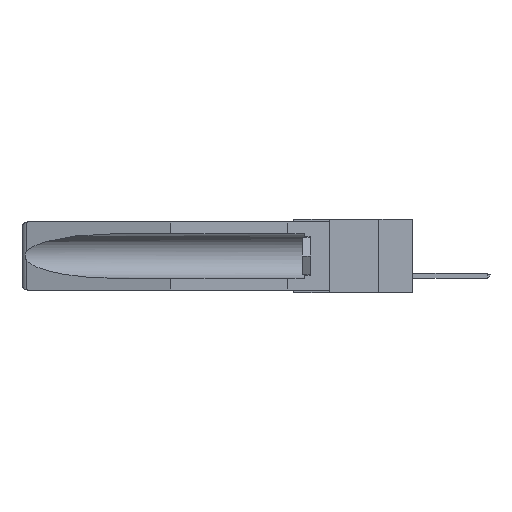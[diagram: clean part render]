
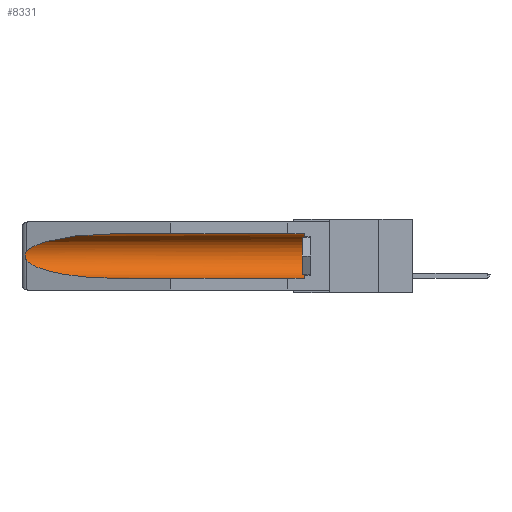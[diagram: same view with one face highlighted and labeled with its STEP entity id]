
A CAD part, left-side view. The second image highlights one B-rep face of the part: STEP entity #8331.
In plain terms, the highlighted cylindrical face has radius 2.857 mm (diameter 5.715 mm), a partial arc.
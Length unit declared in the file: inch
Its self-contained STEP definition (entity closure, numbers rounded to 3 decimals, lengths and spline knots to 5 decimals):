
#1018 = CARTESIAN_POINT ( 'NONE',  ( 0.155, 0.126, -0.284 ) ) ;
#1544 =( BOUNDED_CURVE ( )  B_SPLINE_CURVE ( 3, ( #12412, #15282, #9907, #25426 ),
 .UNSPECIFIED., .F., .F. ) 
 B_SPLINE_CURVE_WITH_KNOTS ( ( 4, 4 ),
 ( 0.1948, 1.5708 ),
 .UNSPECIFIED. ) 
 CURVE ( )  GEOMETRIC_REPRESENTATION_ITEM ( )  RATIONAL_B_SPLINE_CURVE ( ( 1., 0.848, 0.848, 1. ) ) 
 REPRESENTATION_ITEM ( '' )  );
#1725 = CARTESIAN_POINT ( 'NONE',  ( 0.26537, 1.52718, -0.14972 ) ) ;
#3282 = CYLINDRICAL_SURFACE ( 'NONE', #5432, 0.1125 ) ;
#3597 = VERTEX_POINT ( 'NONE', #26638 ) ;
#4484 = DIRECTION ( 'NONE',  ( 0., 0., 1. ) ) ;
#4537 = CARTESIAN_POINT ( 'NONE',  ( 0.2673, 1.5327, -0.16383 ) ) ;
#5125 = VERTEX_POINT ( 'NONE', #1018 ) ;
#5432 = AXIS2_PLACEMENT_3D ( 'NONE', #12078, #9359, #4484 ) ;
#6015 = ORIENTED_EDGE ( 'NONE', *, *, #29916, .T. ) ;
#6448 = CARTESIAN_POINT ( 'NONE',  ( 0.26537, 1.52718, -0.19328 ) ) ;
#7262 = CIRCLE ( 'NONE', #9602, 0.1125 ) ;
#8078 = LINE ( 'NONE', #31128, #20092 ) ;
#8331 = ADVANCED_FACE ( 'NONE', ( #16072 ), #3282, .F. ) ;
#8594 = VERTEX_POINT ( 'NONE', #15827 ) ;
#8678 = EDGE_LOOP ( 'NONE', ( #13634, #25850, #21183, #23184, #6015, #9770 ) ) ;
#9359 = DIRECTION ( 'NONE',  ( 0., 1., 0. ) ) ;
#9602 = AXIS2_PLACEMENT_3D ( 'NONE', #24450, #14224, #14333 ) ;
#9770 = ORIENTED_EDGE ( 'NONE', *, *, #11382, .T. ) ;
#9907 = CARTESIAN_POINT ( 'NONE',  ( 0.21114, 1.30732, -0.284 ) ) ;
#10017 = VERTEX_POINT ( 'NONE', #33198 ) ;
#11382 = EDGE_CURVE ( 'NONE', #27803, #10017, #25628, .T. ) ;
#12078 = CARTESIAN_POINT ( 'NONE',  ( 0.155, -0.30754, -0.1715 ) ) ;
#12137 = CARTESIAN_POINT ( 'NONE',  ( 0.2675, 1.53308, -0.16763 ) ) ;
#12375 = VERTEX_POINT ( 'NONE', #6448 ) ;
#12412 = CARTESIAN_POINT ( 'NONE',  ( 0.26537, 1.52718, -0.19328 ) ) ;
#13436 = B_SPLINE_CURVE_WITH_KNOTS ( 'NONE', 3,
 ( #14808, #30230, #30015, #4537, #12137, #32664, #17392, #27834, #27730, #17497 ),
 .UNSPECIFIED., .F., .F.,
 ( 4, 2, 2, 2, 4 ),
 ( 0., 0.00029, 0.00058, 0.00087, 0.00117 ),
 .UNSPECIFIED. ) ;
#13634 = ORIENTED_EDGE ( 'NONE', *, *, #18317, .T. ) ;
#14224 = DIRECTION ( 'NONE',  ( 0., -1., 0. ) ) ;
#14333 = DIRECTION ( 'NONE',  ( 0., 0., 1. ) ) ;
#14808 = CARTESIAN_POINT ( 'NONE',  ( 0.26537, 1.52718, -0.14972 ) ) ;
#15282 = CARTESIAN_POINT ( 'NONE',  ( 0.25451, 1.48313, -0.24835 ) ) ;
#15570 = CARTESIAN_POINT ( 'NONE',  ( 0.155, 1.07973, -0.059 ) ) ;
#15827 = CARTESIAN_POINT ( 'NONE',  ( 0.26537, 1.52718, -0.14972 ) ) ;
#15932 = EDGE_CURVE ( 'NONE', #5125, #3597, #8078, .T. ) ;
#16072 = FACE_OUTER_BOUND ( 'NONE', #8678, .T. ) ;
#16167 = DIRECTION ( 'NONE',  ( 0., 1., 0. ) ) ;
#16656 = DIRECTION ( 'NONE',  ( 0., 1., 0. ) ) ;
#17167 = CARTESIAN_POINT ( 'NONE',  ( 0.25451, 1.48313, -0.09465 ) ) ;
#17392 = CARTESIAN_POINT ( 'NONE',  ( 0.2673, 1.53269, -0.17917 ) ) ;
#17497 = CARTESIAN_POINT ( 'NONE',  ( 0.26537, 1.52718, -0.19328 ) ) ;
#17944 =( BOUNDED_CURVE ( )  B_SPLINE_CURVE ( 3, ( #15570, #32447, #17167, #1725 ),
 .UNSPECIFIED., .F., .F. ) 
 B_SPLINE_CURVE_WITH_KNOTS ( ( 4, 4 ),
 ( 4.71239, 6.08839 ),
 .UNSPECIFIED. ) 
 CURVE ( )  GEOMETRIC_REPRESENTATION_ITEM ( )  RATIONAL_B_SPLINE_CURVE ( ( 1., 0.848, 0.848, 1. ) ) 
 REPRESENTATION_ITEM ( '' )  );
#18317 = EDGE_CURVE ( 'NONE', #10017, #8594, #17944, .T. ) ;
#18669 = EDGE_CURVE ( 'NONE', #12375, #3597, #1544, .T. ) ;
#20092 = VECTOR ( 'NONE', #16167, 39.37008 ) ;
#21183 = ORIENTED_EDGE ( 'NONE', *, *, #18669, .T. ) ;
#23184 = ORIENTED_EDGE ( 'NONE', *, *, #15932, .F. ) ;
#23199 = VECTOR ( 'NONE', #16656, 39.37008 ) ;
#24450 = CARTESIAN_POINT ( 'NONE',  ( 0.155, 0.126, -0.1715 ) ) ;
#24560 = CARTESIAN_POINT ( 'NONE',  ( 0.155, -0.30754, -0.059 ) ) ;
#25149 = CARTESIAN_POINT ( 'NONE',  ( 0.155, 0.126, -0.059 ) ) ;
#25426 = CARTESIAN_POINT ( 'NONE',  ( 0.155, 1.07973, -0.284 ) ) ;
#25628 = LINE ( 'NONE', #24560, #23199 ) ;
#25850 = ORIENTED_EDGE ( 'NONE', *, *, #31322, .T. ) ;
#26638 = CARTESIAN_POINT ( 'NONE',  ( 0.155, 1.07973, -0.284 ) ) ;
#27730 = CARTESIAN_POINT ( 'NONE',  ( 0.26597, 1.5296, -0.19026 ) ) ;
#27803 = VERTEX_POINT ( 'NONE', #25149 ) ;
#27834 = CARTESIAN_POINT ( 'NONE',  ( 0.26655, 1.53094, -0.18657 ) ) ;
#29916 = EDGE_CURVE ( 'NONE', #5125, #27803, #7262, .T. ) ;
#30015 = CARTESIAN_POINT ( 'NONE',  ( 0.26654, 1.53092, -0.15636 ) ) ;
#30230 = CARTESIAN_POINT ( 'NONE',  ( 0.26597, 1.52961, -0.15275 ) ) ;
#31128 = CARTESIAN_POINT ( 'NONE',  ( 0.155, -0.30754, -0.284 ) ) ;
#31322 = EDGE_CURVE ( 'NONE', #8594, #12375, #13436, .T. ) ;
#32447 = CARTESIAN_POINT ( 'NONE',  ( 0.21114, 1.30732, -0.059 ) ) ;
#32664 = CARTESIAN_POINT ( 'NONE',  ( 0.2675, 1.53308, -0.17534 ) ) ;
#33198 = CARTESIAN_POINT ( 'NONE',  ( 0.155, 1.07973, -0.059 ) ) ;
